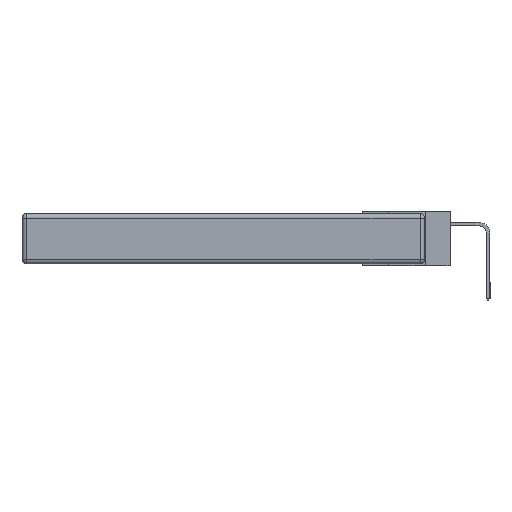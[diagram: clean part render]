
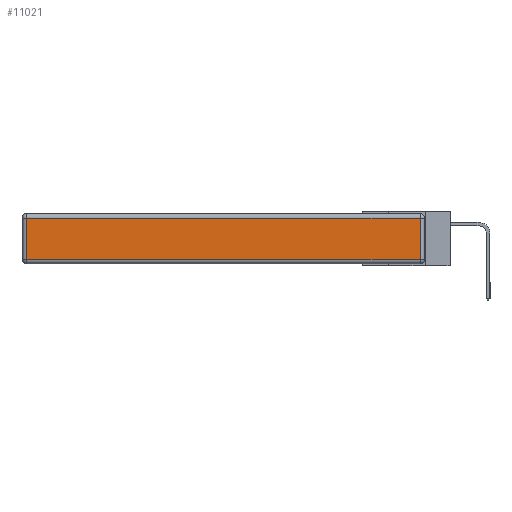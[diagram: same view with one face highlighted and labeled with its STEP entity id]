
A CAD part, left-side view. The second image highlights one B-rep face of the part: STEP entity #11021.
In plain terms, the highlighted planar face has unit normal (-1, 0, 0).
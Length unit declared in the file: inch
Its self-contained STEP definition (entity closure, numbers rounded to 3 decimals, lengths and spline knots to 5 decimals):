
#288 = CARTESIAN_POINT ( 'NONE',  ( 0., 2.72, -0.343 ) ) ;
#717 = ORIENTED_EDGE ( 'NONE', *, *, #10185, .T. ) ;
#814 = CARTESIAN_POINT ( 'NONE',  ( 0., 0., -0.343 ) ) ;
#1029 = EDGE_CURVE ( 'NONE', #4034, #6252, #11792, .T. ) ;
#1464 = CARTESIAN_POINT ( 'NONE',  ( 0., 0.03, -0.343 ) ) ;
#1470 = DIRECTION ( 'NONE',  ( 0., 0., -1. ) ) ;
#2444 = LINE ( 'NONE', #288, #11783 ) ;
#2459 = VECTOR ( 'NONE', #11557, 39.37008 ) ;
#2500 = EDGE_CURVE ( 'NONE', #5286, #4034, #12800, .T. ) ;
#2922 = CARTESIAN_POINT ( 'NONE',  ( 0., 2.75, -0.03 ) ) ;
#4034 = VERTEX_POINT ( 'NONE', #9972 ) ;
#4326 = VERTEX_POINT ( 'NONE', #7734 ) ;
#4381 = CARTESIAN_POINT ( 'NONE',  ( 0., 2.72, -0.313 ) ) ;
#5286 = VERTEX_POINT ( 'NONE', #4381 ) ;
#5434 = CARTESIAN_POINT ( 'NONE',  ( 0., 0., -0.313 ) ) ;
#5574 = DIRECTION ( 'NONE',  ( 0., -1., 0. ) ) ;
#6252 = VERTEX_POINT ( 'NONE', #12419 ) ;
#7734 = CARTESIAN_POINT ( 'NONE',  ( 0., 2.72, -0.03 ) ) ;
#8107 = AXIS2_PLACEMENT_3D ( 'NONE', #814, #10948, #12077 ) ;
#8941 = EDGE_LOOP ( 'NONE', ( #13002, #10967, #717, #10293 ) ) ;
#9315 = FACE_OUTER_BOUND ( 'NONE', #8941, .T. ) ;
#9672 = LINE ( 'NONE', #2922, #11954 ) ;
#9694 = DIRECTION ( 'NONE',  ( 0., 1., 0. ) ) ;
#9860 = PLANE ( 'NONE',  #8107 ) ;
#9972 = CARTESIAN_POINT ( 'NONE',  ( 0., 0.03, -0.313 ) ) ;
#10185 = EDGE_CURVE ( 'NONE', #6252, #4326, #9672, .T. ) ;
#10293 = ORIENTED_EDGE ( 'NONE', *, *, #13431, .T. ) ;
#10948 = DIRECTION ( 'NONE',  ( -1., 0., 0. ) ) ;
#10967 = ORIENTED_EDGE ( 'NONE', *, *, #1029, .T. ) ;
#11021 = ADVANCED_FACE ( 'NONE', ( #9315 ), #9860, .T. ) ;
#11557 = DIRECTION ( 'NONE',  ( 0., 0., 1. ) ) ;
#11783 = VECTOR ( 'NONE', #1470, 39.37008 ) ;
#11792 = LINE ( 'NONE', #1464, #2459 ) ;
#11954 = VECTOR ( 'NONE', #9694, 39.37008 ) ;
#12077 = DIRECTION ( 'NONE',  ( 0., 0., 1. ) ) ;
#12419 = CARTESIAN_POINT ( 'NONE',  ( 0., 0.03, -0.03 ) ) ;
#12618 = VECTOR ( 'NONE', #5574, 39.37008 ) ;
#12800 = LINE ( 'NONE', #5434, #12618 ) ;
#13002 = ORIENTED_EDGE ( 'NONE', *, *, #2500, .T. ) ;
#13431 = EDGE_CURVE ( 'NONE', #4326, #5286, #2444, .T. ) ;
